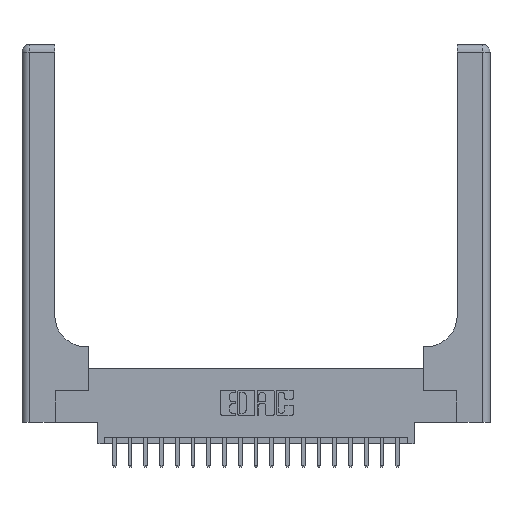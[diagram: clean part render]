
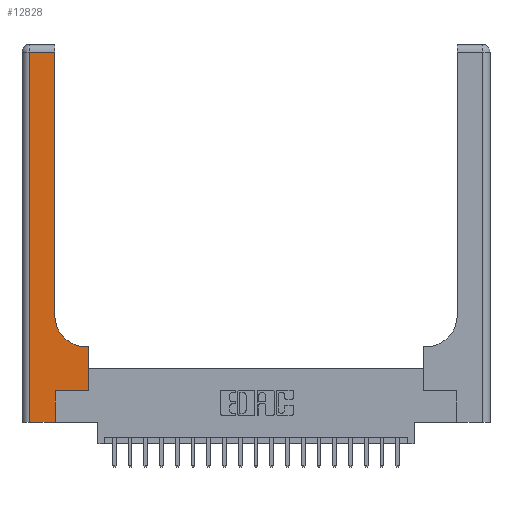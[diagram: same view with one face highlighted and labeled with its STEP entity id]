
A CAD part, top view. The second image highlights one B-rep face of the part: STEP entity #12828.
In plain terms, the highlighted planar face has unit normal (0, 0, 1).
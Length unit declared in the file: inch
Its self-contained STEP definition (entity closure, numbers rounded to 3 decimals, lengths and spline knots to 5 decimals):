
#491 = VECTOR ( 'NONE', #4393, 39.37008 ) ;
#549 = DIRECTION ( 'NONE',  ( -1., 0., 0. ) ) ;
#555 = CARTESIAN_POINT ( 'NONE',  ( 0.26, 0.6, 0.37 ) ) ;
#617 = LINE ( 'NONE', #7340, #9504 ) ;
#833 = VECTOR ( 'NONE', #12102, 39.37008 ) ;
#877 = CARTESIAN_POINT ( 'NONE',  ( 0.26, 0.85, 0.37 ) ) ;
#1320 = CARTESIAN_POINT ( 'NONE',  ( 0.528, 0.6, 0.37 ) ) ;
#1645 = EDGE_CURVE ( 'NONE', #10085, #3240, #13248, .T. ) ;
#1854 = ORIENTED_EDGE ( 'NONE', *, *, #3048, .T. ) ;
#3048 = EDGE_CURVE ( 'NONE', #13469, #19712, #16412, .T. ) ;
#3098 = CARTESIAN_POINT ( 'NONE',  ( 0., 3., 0.37 ) ) ;
#3190 = EDGE_CURVE ( 'NONE', #3240, #5737, #13598, .T. ) ;
#3240 = VERTEX_POINT ( 'NONE', #13502 ) ;
#3891 = CARTESIAN_POINT ( 'NONE',  ( 0.51, 0.85, 0.37 ) ) ;
#3952 = CARTESIAN_POINT ( 'NONE',  ( 0.06, 2.94, 0.37 ) ) ;
#4266 = EDGE_CURVE ( 'NONE', #19712, #6612, #20748, .T. ) ;
#4286 = VERTEX_POINT ( 'NONE', #6185 ) ;
#4290 = DIRECTION ( 'NONE',  ( 0., 1., 0. ) ) ;
#4393 = DIRECTION ( 'NONE',  ( 1., 0., 0. ) ) ;
#5737 = VERTEX_POINT ( 'NONE', #1320 ) ;
#6185 = CARTESIAN_POINT ( 'NONE',  ( 0.51, 0.6, 0.37 ) ) ;
#6351 = ORIENTED_EDGE ( 'NONE', *, *, #11926, .T. ) ;
#6612 = VERTEX_POINT ( 'NONE', #3952 ) ;
#6938 = VECTOR ( 'NONE', #19816, 39.37008 ) ;
#7005 = ORIENTED_EDGE ( 'NONE', *, *, #8725, .T. ) ;
#7156 = DIRECTION ( 'NONE',  ( 0., 0., -1. ) ) ;
#7340 = CARTESIAN_POINT ( 'NONE',  ( 0.265, 0., 0.37 ) ) ;
#7640 = ORIENTED_EDGE ( 'NONE', *, *, #14959, .T. ) ;
#7701 = VERTEX_POINT ( 'NONE', #12453 ) ;
#7849 = ORIENTED_EDGE ( 'NONE', *, *, #15614, .T. ) ;
#8181 = CARTESIAN_POINT ( 'NONE',  ( 0.265, 0.25, 0.37 ) ) ;
#8725 = EDGE_CURVE ( 'NONE', #5737, #4286, #11819, .T. ) ;
#9055 = CARTESIAN_POINT ( 'NONE',  ( 0., 0., 0.37 ) ) ;
#9504 = VECTOR ( 'NONE', #4290, 39.37008 ) ;
#9612 = ORIENTED_EDGE ( 'NONE', *, *, #3190, .T. ) ;
#9940 = ORIENTED_EDGE ( 'NONE', *, *, #4266, .T. ) ;
#10085 = VERTEX_POINT ( 'NONE', #13430 ) ;
#10089 = ORIENTED_EDGE ( 'NONE', *, *, #10187, .T. ) ;
#10167 = CIRCLE ( 'NONE', #16039, 0.25 ) ;
#10187 = EDGE_CURVE ( 'NONE', #6612, #7701, #11134, .T. ) ;
#10710 = CARTESIAN_POINT ( 'NONE',  ( 0.06, 3., 0.37 ) ) ;
#11134 = LINE ( 'NONE', #10710, #20393 ) ;
#11626 = DIRECTION ( 'NONE',  ( -1., 0., 0. ) ) ;
#11819 = LINE ( 'NONE', #555, #17557 ) ;
#11926 = EDGE_CURVE ( 'NONE', #7701, #20405, #19075, .T. ) ;
#12102 = DIRECTION ( 'NONE',  ( 0., 1., 0. ) ) ;
#12453 = CARTESIAN_POINT ( 'NONE',  ( 0.06, 0., 0.37 ) ) ;
#12458 = EDGE_LOOP ( 'NONE', ( #1854, #9940, #10089, #6351, #7849, #20561, #9612, #7005, #7640 ) ) ;
#12551 = CARTESIAN_POINT ( 'NONE',  ( 0., 2.94, 0.37 ) ) ;
#12828 = ADVANCED_FACE ( 'NONE', ( #19916 ), #12919, .F. ) ;
#12919 = PLANE ( 'NONE',  #16568 ) ;
#13248 = LINE ( 'NONE', #8181, #6938 ) ;
#13430 = CARTESIAN_POINT ( 'NONE',  ( 0.265, 0.25, 0.37 ) ) ;
#13469 = VERTEX_POINT ( 'NONE', #877 ) ;
#13502 = CARTESIAN_POINT ( 'NONE',  ( 0.528, 0.25, 0.37 ) ) ;
#13522 = DIRECTION ( 'NONE',  ( 1., 0., 0. ) ) ;
#13598 = LINE ( 'NONE', #16949, #833 ) ;
#14050 = DIRECTION ( 'NONE',  ( 0., -1., 0. ) ) ;
#14761 = DIRECTION ( 'NONE',  ( 0., 0., -1. ) ) ;
#14796 = DIRECTION ( 'NONE',  ( 0., 1., 0. ) ) ;
#14959 = EDGE_CURVE ( 'NONE', #4286, #13469, #10167, .T. ) ;
#15614 = EDGE_CURVE ( 'NONE', #20405, #10085, #617, .T. ) ;
#15681 = VECTOR ( 'NONE', #14796, 39.37008 ) ;
#16039 = AXIS2_PLACEMENT_3D ( 'NONE', #3891, #7156, #13522 ) ;
#16412 = LINE ( 'NONE', #21070, #15681 ) ;
#16568 = AXIS2_PLACEMENT_3D ( 'NONE', #3098, #14761, #11626 ) ;
#16696 = VECTOR ( 'NONE', #549, 39.37008 ) ;
#16949 = CARTESIAN_POINT ( 'NONE',  ( 0.528, 0.25, 0.37 ) ) ;
#17557 = VECTOR ( 'NONE', #18585, 39.37008 ) ;
#17892 = CARTESIAN_POINT ( 'NONE',  ( 0.265, 0., 0.37 ) ) ;
#18585 = DIRECTION ( 'NONE',  ( -1., 0., 0. ) ) ;
#19075 = LINE ( 'NONE', #9055, #491 ) ;
#19712 = VERTEX_POINT ( 'NONE', #20817 ) ;
#19816 = DIRECTION ( 'NONE',  ( 1., 0., 0. ) ) ;
#19916 = FACE_OUTER_BOUND ( 'NONE', #12458, .T. ) ;
#20393 = VECTOR ( 'NONE', #14050, 39.37008 ) ;
#20405 = VERTEX_POINT ( 'NONE', #17892 ) ;
#20561 = ORIENTED_EDGE ( 'NONE', *, *, #1645, .T. ) ;
#20748 = LINE ( 'NONE', #12551, #16696 ) ;
#20817 = CARTESIAN_POINT ( 'NONE',  ( 0.26, 2.94, 0.37 ) ) ;
#21070 = CARTESIAN_POINT ( 'NONE',  ( 0.26, 3., 0.37 ) ) ;
